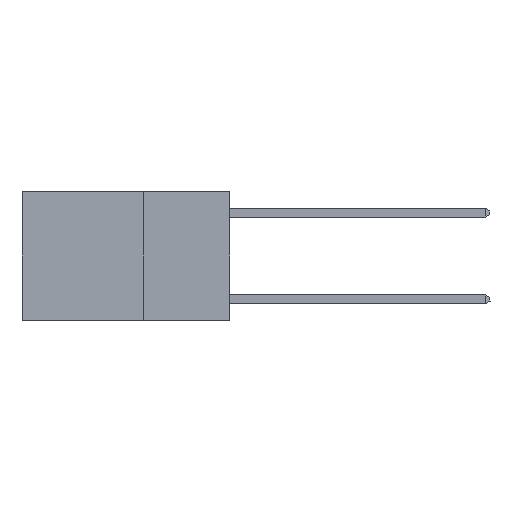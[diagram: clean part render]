
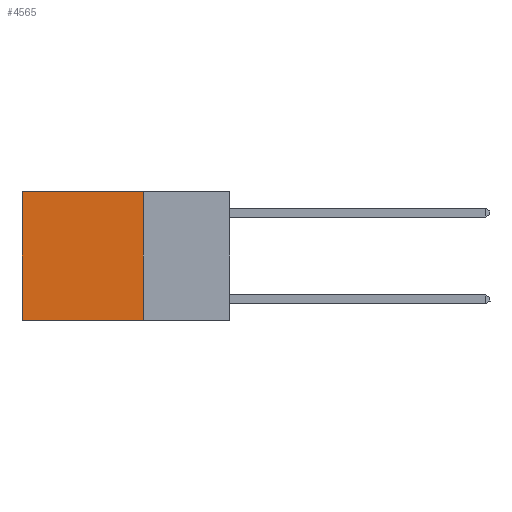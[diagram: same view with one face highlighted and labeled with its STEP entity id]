
A CAD part, left-side view. The second image highlights one B-rep face of the part: STEP entity #4565.
In plain terms, the highlighted planar face has unit normal (-1, 0, 0).
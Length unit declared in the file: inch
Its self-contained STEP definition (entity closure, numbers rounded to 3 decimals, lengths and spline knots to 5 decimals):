
#698 = ORIENTED_EDGE ( 'NONE', *, *, #8642, .F. ) ;
#911 = CARTESIAN_POINT ( 'NONE',  ( 0.2625, 0.25, 0. ) ) ;
#1924 = DIRECTION ( 'NONE',  ( 0., 0., -1. ) ) ;
#2115 = DIRECTION ( 'NONE',  ( 0., 0., -1. ) ) ;
#2118 = DIRECTION ( 'NONE',  ( 0., 1., 0. ) ) ;
#2790 = CARTESIAN_POINT ( 'NONE',  ( 0.2625, 0.25, 0. ) ) ;
#3409 = EDGE_CURVE ( 'NONE', #6554, #5089, #7665, .T. ) ;
#4170 = FACE_OUTER_BOUND ( 'NONE', #13790, .T. ) ;
#4330 = PLANE ( 'NONE',  #10033 ) ;
#4565 = ADVANCED_FACE ( 'NONE', ( #4170 ), #4330, .F. ) ;
#4994 = VERTEX_POINT ( 'NONE', #2790 ) ;
#5089 = VERTEX_POINT ( 'NONE', #13073 ) ;
#5459 = CARTESIAN_POINT ( 'NONE',  ( 0.2625, 0.25, 0. ) ) ;
#5796 = VERTEX_POINT ( 'NONE', #11529 ) ;
#6027 = DIRECTION ( 'NONE',  ( 0., 0., -1. ) ) ;
#6164 = ORIENTED_EDGE ( 'NONE', *, *, #3409, .F. ) ;
#6554 = VERTEX_POINT ( 'NONE', #12955 ) ;
#6861 = CARTESIAN_POINT ( 'NONE',  ( 0.2625, 0.25, -0.37 ) ) ;
#7665 = LINE ( 'NONE', #6861, #13673 ) ;
#7698 = EDGE_CURVE ( 'NONE', #5796, #5089, #11080, .T. ) ;
#7722 = VECTOR ( 'NONE', #6027, 39.37008 ) ;
#8099 = LINE ( 'NONE', #911, #10739 ) ;
#8194 = CARTESIAN_POINT ( 'NONE',  ( 0.2625, 0.6, 0. ) ) ;
#8642 = EDGE_CURVE ( 'NONE', #4994, #6554, #8905, .T. ) ;
#8801 = DIRECTION ( 'NONE',  ( 1., 0., 0. ) ) ;
#8905 = LINE ( 'NONE', #9733, #11964 ) ;
#9067 = DIRECTION ( 'NONE',  ( 0., 1., 0. ) ) ;
#9733 = CARTESIAN_POINT ( 'NONE',  ( 0.2625, 0.25, 0. ) ) ;
#10033 = AXIS2_PLACEMENT_3D ( 'NONE', #5459, #8801, #2115 ) ;
#10739 = VECTOR ( 'NONE', #2118, 39.37008 ) ;
#11080 = LINE ( 'NONE', #8194, #7722 ) ;
#11235 = ORIENTED_EDGE ( 'NONE', *, *, #7698, .T. ) ;
#11529 = CARTESIAN_POINT ( 'NONE',  ( 0.2625, 0.6, 0. ) ) ;
#11964 = VECTOR ( 'NONE', #1924, 39.37008 ) ;
#12440 = EDGE_CURVE ( 'NONE', #4994, #5796, #8099, .T. ) ;
#12955 = CARTESIAN_POINT ( 'NONE',  ( 0.2625, 0.25, -0.37 ) ) ;
#13073 = CARTESIAN_POINT ( 'NONE',  ( 0.2625, 0.6, -0.37 ) ) ;
#13178 = ORIENTED_EDGE ( 'NONE', *, *, #12440, .T. ) ;
#13673 = VECTOR ( 'NONE', #9067, 39.37008 ) ;
#13790 = EDGE_LOOP ( 'NONE', ( #11235, #6164, #698, #13178 ) ) ;
